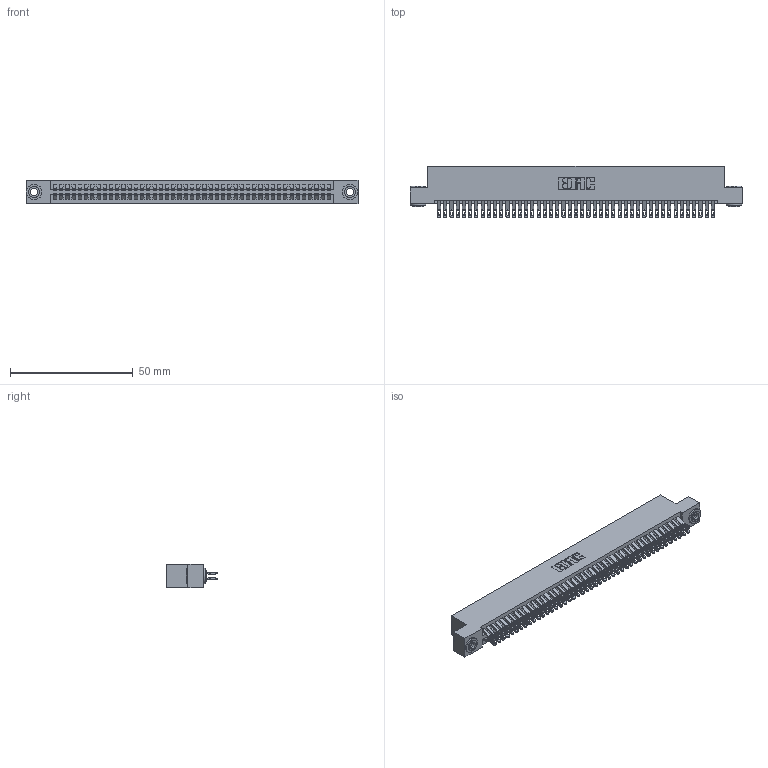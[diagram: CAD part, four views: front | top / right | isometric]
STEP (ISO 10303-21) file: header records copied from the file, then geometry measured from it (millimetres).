
FILE_DESCRIPTION (( 'STEP AP203' ), '1' );
FILE_NAME ('395-090-555-203.STEP', '2018-11-29T04:32:10', ( '' ), ( '' ), 'SwSTEP 2.0', 'SolidWorks 2016', '' );
FILE_SCHEMA (( 'CONFIG_CONTROL_DESIGN' ));
Length unit declared in the file: inch
Products named in the file (4): 345-250-002_345-250-002-102; 345-292-001_555 Tail; 395-090-555-203; 345 Part_Flush Mounting Lugs - 0.156 Dia-TH
Assembly tree (93 placements, depth 2):
  395-090-555-203
    345 Part_Flush Mounting Lugs - 0.156 Dia-TH
    345-292-001_555 Tail  x90
    345-250-002_345-250-002-102  x2
Bounding box: 135.51 x 21.13 x 9.4 mm (x, y, z)
Volume: 13471.8 mm3; surface area: 21084.5 mm2
Topology: 93 solids, 93 shells, 5204 faces, 16347 edges, 10894 vertices
Faces by surface type: plane 2880, cylinder 2316, cone 8
Entity records: 35880 total; most frequent: CARTESIAN_POINT 6021, ORIENTED_EDGE 5918, DIRECTION 5305, EDGE_CURVE 2959, VECTOR 2603, LINE 2603, VERTEX_POINT 1970, AXIS2_PLACEMENT_3D 1351
